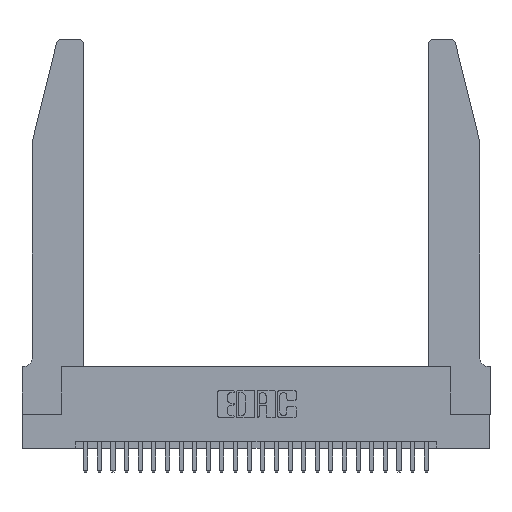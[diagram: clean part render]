
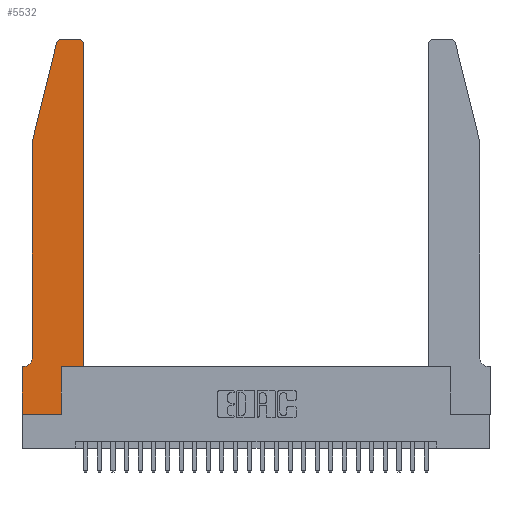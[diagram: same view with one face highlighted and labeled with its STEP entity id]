
A CAD part, top view. The second image highlights one B-rep face of the part: STEP entity #5532.
In plain terms, the highlighted planar face has unit normal (0, 0, 1).
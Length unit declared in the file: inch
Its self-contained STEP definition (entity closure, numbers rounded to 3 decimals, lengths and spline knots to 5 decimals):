
#86 = CARTESIAN_POINT ( 'NONE',  ( 0.25487, 2.72718, 0.37 ) ) ;
#313 = DIRECTION ( 'NONE',  ( -1., 0., 0. ) ) ;
#549 = LINE ( 'NONE', #4534, #5586 ) ;
#652 = CARTESIAN_POINT ( 'NONE',  ( 0., 0.35, 0.37 ) ) ;
#762 = EDGE_CURVE ( 'NONE', #15945, #15382, #1869, .T. ) ;
#819 = DIRECTION ( 'NONE',  ( 1., 0., 0. ) ) ;
#942 = EDGE_CURVE ( 'NONE', #3193, #7843, #2185, .T. ) ;
#1188 = VECTOR ( 'NONE', #9976, 39.37008 ) ;
#1587 = ORIENTED_EDGE ( 'NONE', *, *, #9461, .T. ) ;
#1869 = LINE ( 'NONE', #11900, #1188 ) ;
#2185 = CIRCLE ( 'NONE', #24993, 0.03 ) ;
#2240 = CARTESIAN_POINT ( 'NONE',  ( 0.4505, 2.72, 0.37 ) ) ;
#2422 = CARTESIAN_POINT ( 'NONE',  ( 0.4205, 2.75, 0.37 ) ) ;
#2804 = DIRECTION ( 'NONE',  ( 0., 0., 1. ) ) ;
#3193 = VERTEX_POINT ( 'NONE', #23255 ) ;
#3651 = ORIENTED_EDGE ( 'NONE', *, *, #13073, .T. ) ;
#3794 = EDGE_CURVE ( 'NONE', #19040, #16491, #24356, .T. ) ;
#4534 = CARTESIAN_POINT ( 'NONE',  ( 0., 0., 0.37 ) ) ;
#4684 = CARTESIAN_POINT ( 'NONE',  ( 0., 0., 0.37 ) ) ;
#4857 = AXIS2_PLACEMENT_3D ( 'NONE', #652, #2804, #17738 ) ;
#4963 = AXIS2_PLACEMENT_3D ( 'NONE', #6688, #21530, #8834 ) ;
#5382 = VERTEX_POINT ( 'NONE', #23500 ) ;
#5532 = ADVANCED_FACE ( 'NONE', ( #22647 ), #13456, .T. ) ;
#5586 = VECTOR ( 'NONE', #6571, 39.37008 ) ;
#5829 = CARTESIAN_POINT ( 'NONE',  ( 0., 0.35, 0.37 ) ) ;
#6230 = VECTOR ( 'NONE', #6603, 39.37008 ) ;
#6571 = DIRECTION ( 'NONE',  ( 1., 0., 0. ) ) ;
#6603 = DIRECTION ( 'NONE',  ( 0., -1., 0. ) ) ;
#6645 = CIRCLE ( 'NONE', #13706, 0.07 ) ;
#6688 = CARTESIAN_POINT ( 'NONE',  ( 0.4205, 2.72, 0.37 ) ) ;
#6805 = DIRECTION ( 'NONE',  ( 0., -1., 0. ) ) ;
#6882 = VECTOR ( 'NONE', #6805, 39.37008 ) ;
#7099 = CARTESIAN_POINT ( 'NONE',  ( 0.0755, 0.42, 0.37 ) ) ;
#7700 = VERTEX_POINT ( 'NONE', #2422 ) ;
#7843 = VERTEX_POINT ( 'NONE', #86 ) ;
#8043 = VERTEX_POINT ( 'NONE', #7099 ) ;
#8834 = DIRECTION ( 'NONE',  ( 1., 0., 0. ) ) ;
#9045 = ORIENTED_EDGE ( 'NONE', *, *, #11976, .T. ) ;
#9179 = ORIENTED_EDGE ( 'NONE', *, *, #3794, .T. ) ;
#9325 = CIRCLE ( 'NONE', #4963, 0.03 ) ;
#9461 = EDGE_CURVE ( 'NONE', #7843, #13743, #24042, .T. ) ;
#9976 = DIRECTION ( 'NONE',  ( 0., 1., 0. ) ) ;
#10711 = LINE ( 'NONE', #11477, #16394 ) ;
#11012 = CARTESIAN_POINT ( 'NONE',  ( 0.0755, 0.35, 0.37 ) ) ;
#11477 = CARTESIAN_POINT ( 'NONE',  ( 0.4505, 0.35, 0.37 ) ) ;
#11604 = LINE ( 'NONE', #25093, #16600 ) ;
#11900 = CARTESIAN_POINT ( 'NONE',  ( 0.4505, 0.35, 0.37 ) ) ;
#11976 = EDGE_CURVE ( 'NONE', #16491, #15945, #10711, .T. ) ;
#12668 = EDGE_LOOP ( 'NONE', ( #23657, #15514, #1587, #17627, #3651, #23633, #19885, #26615, #9179, #9045, #21973, #15308 ) ) ;
#12823 = VECTOR ( 'NONE', #20489, 39.37008 ) ;
#13073 = EDGE_CURVE ( 'NONE', #8043, #17132, #6645, .T. ) ;
#13101 = DIRECTION ( 'NONE',  ( 0., 0., -1. ) ) ;
#13456 = PLANE ( 'NONE',  #4857 ) ;
#13706 = AXIS2_PLACEMENT_3D ( 'NONE', #25721, #13101, #313 ) ;
#13743 = VERTEX_POINT ( 'NONE', #21920 ) ;
#14097 = EDGE_CURVE ( 'NONE', #7700, #3193, #11604, .T. ) ;
#14496 = VECTOR ( 'NONE', #25526, 39.37008 ) ;
#14631 = VERTEX_POINT ( 'NONE', #5829 ) ;
#15025 = CARTESIAN_POINT ( 'NONE',  ( 0.2865, 0., 0.37 ) ) ;
#15288 = CARTESIAN_POINT ( 'NONE',  ( 0.0755, 2., 0.37 ) ) ;
#15308 = ORIENTED_EDGE ( 'NONE', *, *, #24898, .T. ) ;
#15382 = VERTEX_POINT ( 'NONE', #2240 ) ;
#15468 = EDGE_CURVE ( 'NONE', #14631, #5382, #24431, .T. ) ;
#15514 = ORIENTED_EDGE ( 'NONE', *, *, #942, .T. ) ;
#15945 = VERTEX_POINT ( 'NONE', #21073 ) ;
#16394 = VECTOR ( 'NONE', #819, 39.37008 ) ;
#16491 = VERTEX_POINT ( 'NONE', #24973 ) ;
#16600 = VECTOR ( 'NONE', #20901, 39.37008 ) ;
#17132 = VERTEX_POINT ( 'NONE', #25488 ) ;
#17611 = VECTOR ( 'NONE', #25847, 39.37008 ) ;
#17627 = ORIENTED_EDGE ( 'NONE', *, *, #26022, .T. ) ;
#17738 = DIRECTION ( 'NONE',  ( 1., 0., 0. ) ) ;
#19040 = VERTEX_POINT ( 'NONE', #15025 ) ;
#19164 = EDGE_CURVE ( 'NONE', #17132, #14631, #23814, .T. ) ;
#19645 = EDGE_CURVE ( 'NONE', #5382, #19040, #549, .T. ) ;
#19885 = ORIENTED_EDGE ( 'NONE', *, *, #15468, .T. ) ;
#20489 = DIRECTION ( 'NONE',  ( -0.239, -0.971, 0. ) ) ;
#20901 = DIRECTION ( 'NONE',  ( -1., 0., 0. ) ) ;
#21073 = CARTESIAN_POINT ( 'NONE',  ( 0.4505, 0.35, 0.37 ) ) ;
#21324 = CARTESIAN_POINT ( 'NONE',  ( 0.2865, 0.35, 0.37 ) ) ;
#21530 = DIRECTION ( 'NONE',  ( 0., 0., 1. ) ) ;
#21920 = CARTESIAN_POINT ( 'NONE',  ( 0.0755, 2., 0.37 ) ) ;
#21973 = ORIENTED_EDGE ( 'NONE', *, *, #762, .T. ) ;
#22519 = CARTESIAN_POINT ( 'NONE',  ( 0.0755, 2., 0.37 ) ) ;
#22647 = FACE_OUTER_BOUND ( 'NONE', #12668, .T. ) ;
#23255 = CARTESIAN_POINT ( 'NONE',  ( 0.284, 2.75, 0.37 ) ) ;
#23500 = CARTESIAN_POINT ( 'NONE',  ( 0., 0., 0.37 ) ) ;
#23633 = ORIENTED_EDGE ( 'NONE', *, *, #19164, .T. ) ;
#23657 = ORIENTED_EDGE ( 'NONE', *, *, #14097, .T. ) ;
#23785 = LINE ( 'NONE', #15288, #6230 ) ;
#23814 = LINE ( 'NONE', #11012, #17611 ) ;
#23953 = DIRECTION ( 'NONE',  ( 0., 0., 1. ) ) ;
#24042 = LINE ( 'NONE', #22519, #12823 ) ;
#24131 = DIRECTION ( 'NONE',  ( 1., 0., 0. ) ) ;
#24356 = LINE ( 'NONE', #21324, #14496 ) ;
#24431 = LINE ( 'NONE', #4684, #6882 ) ;
#24898 = EDGE_CURVE ( 'NONE', #15382, #7700, #9325, .T. ) ;
#24973 = CARTESIAN_POINT ( 'NONE',  ( 0.2865, 0.35, 0.37 ) ) ;
#24993 = AXIS2_PLACEMENT_3D ( 'NONE', #25531, #23953, #24131 ) ;
#25093 = CARTESIAN_POINT ( 'NONE',  ( 0.2605, 2.75, 0.37 ) ) ;
#25488 = CARTESIAN_POINT ( 'NONE',  ( 0.0055, 0.35, 0.37 ) ) ;
#25526 = DIRECTION ( 'NONE',  ( 0., 1., 0. ) ) ;
#25531 = CARTESIAN_POINT ( 'NONE',  ( 0.284, 2.72, 0.37 ) ) ;
#25721 = CARTESIAN_POINT ( 'NONE',  ( 0.0055, 0.42, 0.37 ) ) ;
#25847 = DIRECTION ( 'NONE',  ( -1., 0., 0. ) ) ;
#26022 = EDGE_CURVE ( 'NONE', #13743, #8043, #23785, .T. ) ;
#26615 = ORIENTED_EDGE ( 'NONE', *, *, #19645, .T. ) ;
